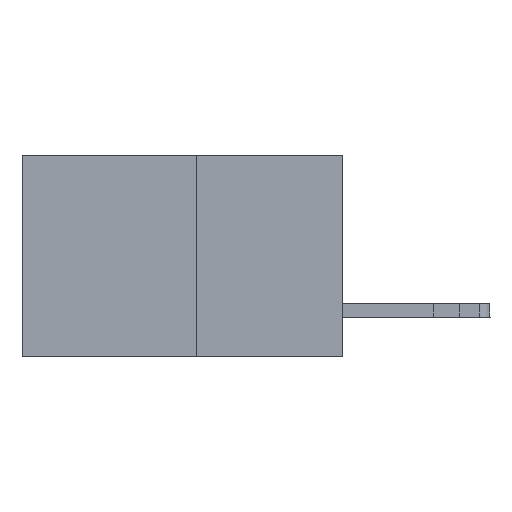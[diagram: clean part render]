
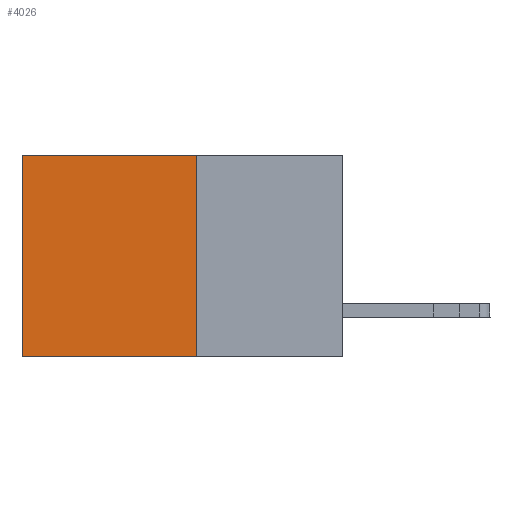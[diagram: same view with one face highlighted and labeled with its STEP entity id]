
A CAD part, left-side view. The second image highlights one B-rep face of the part: STEP entity #4026.
In plain terms, the highlighted planar face has unit normal (-1, 0, 0).
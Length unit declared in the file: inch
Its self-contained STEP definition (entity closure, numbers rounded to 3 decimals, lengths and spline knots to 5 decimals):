
#48 = VERTEX_POINT ( 'NONE', #2840 ) ;
#321 = LINE ( 'NONE', #2675, #15894 ) ;
#672 = DIRECTION ( 'NONE',  ( 0., 0., -1. ) ) ;
#815 = DIRECTION ( 'NONE',  ( 0., 0., -1. ) ) ;
#992 = LINE ( 'NONE', #4572, #8270 ) ;
#1480 = VERTEX_POINT ( 'NONE', #7983 ) ;
#1774 = ORIENTED_EDGE ( 'NONE', *, *, #4314, .T. ) ;
#2071 = CARTESIAN_POINT ( 'NONE',  ( 0.277, 0.59, -0.37 ) ) ;
#2149 = DIRECTION ( 'NONE',  ( 0., 0., -1. ) ) ;
#2675 = CARTESIAN_POINT ( 'NONE',  ( 0.277, 0.27, 0. ) ) ;
#2840 = CARTESIAN_POINT ( 'NONE',  ( 0.277, 0.27, -0.37 ) ) ;
#3948 = VERTEX_POINT ( 'NONE', #5624 ) ;
#4026 = ADVANCED_FACE ( 'NONE', ( #7015 ), #8303, .F. ) ;
#4134 = VERTEX_POINT ( 'NONE', #5950 ) ;
#4314 = EDGE_CURVE ( 'NONE', #1480, #3948, #321, .T. ) ;
#4572 = CARTESIAN_POINT ( 'NONE',  ( 0.277, 0.27, -0.37 ) ) ;
#4927 = ORIENTED_EDGE ( 'NONE', *, *, #9487, .F. ) ;
#5198 = DIRECTION ( 'NONE',  ( 0., 1., 0. ) ) ;
#5624 = CARTESIAN_POINT ( 'NONE',  ( 0.277, 0.59, 0. ) ) ;
#5950 = CARTESIAN_POINT ( 'NONE',  ( 0.277, 0.59, -0.37 ) ) ;
#6807 = LINE ( 'NONE', #2071, #15188 ) ;
#7015 = FACE_OUTER_BOUND ( 'NONE', #9337, .T. ) ;
#7983 = CARTESIAN_POINT ( 'NONE',  ( 0.277, 0.27, 0. ) ) ;
#8270 = VECTOR ( 'NONE', #10907, 39.37008 ) ;
#8303 = PLANE ( 'NONE',  #14844 ) ;
#9090 = ORIENTED_EDGE ( 'NONE', *, *, #15820, .F. ) ;
#9299 = CARTESIAN_POINT ( 'NONE',  ( 0.277, 0.27, -0.37 ) ) ;
#9337 = EDGE_LOOP ( 'NONE', ( #9531, #4927, #9090, #1774 ) ) ;
#9487 = EDGE_CURVE ( 'NONE', #48, #4134, #992, .T. ) ;
#9531 = ORIENTED_EDGE ( 'NONE', *, *, #12210, .T. ) ;
#10666 = CARTESIAN_POINT ( 'NONE',  ( 0.277, 0.27, -0.37 ) ) ;
#10907 = DIRECTION ( 'NONE',  ( 0., 1., 0. ) ) ;
#11977 = DIRECTION ( 'NONE',  ( 1., 0., 0. ) ) ;
#12210 = EDGE_CURVE ( 'NONE', #3948, #4134, #6807, .T. ) ;
#12576 = VECTOR ( 'NONE', #672, 39.37008 ) ;
#14844 = AXIS2_PLACEMENT_3D ( 'NONE', #9299, #11977, #815 ) ;
#15188 = VECTOR ( 'NONE', #2149, 39.37008 ) ;
#15624 = LINE ( 'NONE', #10666, #12576 ) ;
#15820 = EDGE_CURVE ( 'NONE', #1480, #48, #15624, .T. ) ;
#15894 = VECTOR ( 'NONE', #5198, 39.37008 ) ;
